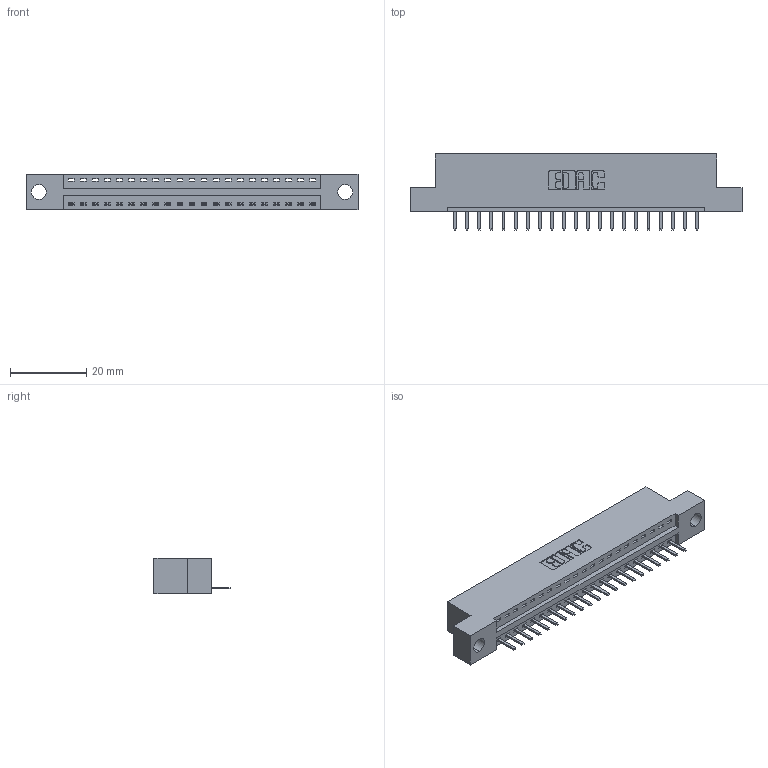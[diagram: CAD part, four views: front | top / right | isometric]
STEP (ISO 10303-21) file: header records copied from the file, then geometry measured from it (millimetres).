
FILE_DESCRIPTION (( 'STEP AP203' ), '1' );
FILE_NAME ('346-021-520-104.STEP', '2018-08-20T22:40:28', ( '' ), ( '' ), 'SwSTEP 2.0', 'SolidWorks 2016', '' );
FILE_SCHEMA (( 'CONFIG_CONTROL_DESIGN' ));
Length unit declared in the file: inch
Products named in the file (3): 346-021-520-104; 346 Part_Flush Mounting Lugs - 0.156 Dia-TH; 345-292-001_345-293-120
Assembly tree (22 placements, depth 2):
  346-021-520-104
    346 Part_Flush Mounting Lugs - 0.156 Dia-TH
    345-292-001_345-293-120  x21
Bounding box: 87.25 x 20.02 x 9.4 mm (x, y, z)
Volume: 8058.7 mm3; surface area: 9449.1 mm2
Topology: 22 solids, 22 shells, 1424 faces, 4193 edges, 2738 vertices
Faces by surface type: plane 958, cylinder 466
Entity records: 15977 total; most frequent: CARTESIAN_POINT 2763, ORIENTED_EDGE 2706, DIRECTION 2451, EDGE_CURVE 1353, VECTOR 1133, LINE 1133, VERTEX_POINT 898, AXIS2_PLACEMENT_3D 659
